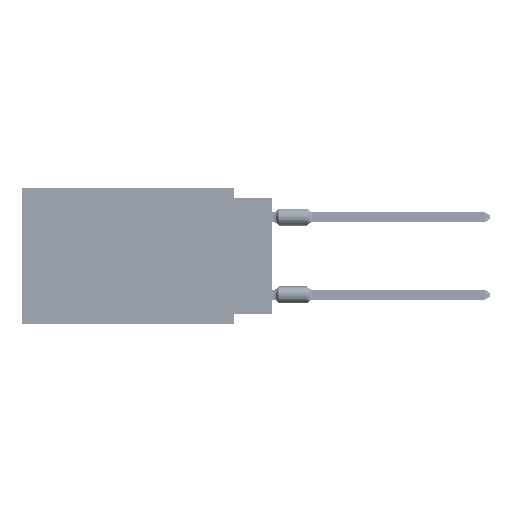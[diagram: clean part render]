
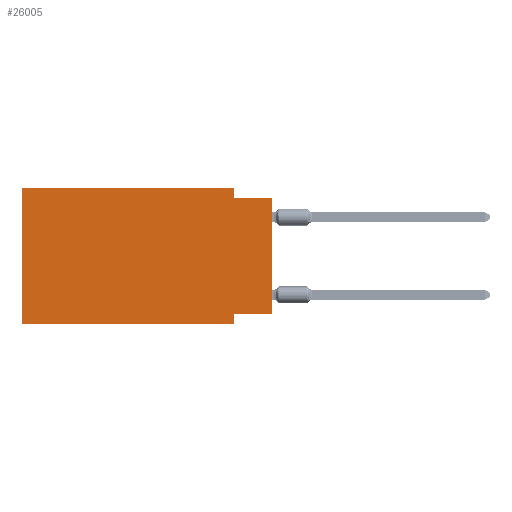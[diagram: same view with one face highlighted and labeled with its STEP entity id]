
A CAD part, left-side view. The second image highlights one B-rep face of the part: STEP entity #26005.
In plain terms, the highlighted planar face has unit normal (-1, 0, 0).
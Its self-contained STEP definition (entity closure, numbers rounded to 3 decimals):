
#1491 = VECTOR ( 'NONE', #83403, 1000. ) ;
#2519 = EDGE_CURVE ( 'NONE', #63819, #56504, #34661, .T. ) ;
#3334 = DIRECTION ( 'NONE',  ( 0., 0., -1. ) ) ;
#5311 = EDGE_CURVE ( 'NONE', #20957, #39904, #30329, .T. ) ;
#7591 = ORIENTED_EDGE ( 'NONE', *, *, #12461, .F. ) ;
#8471 = EDGE_CURVE ( 'NONE', #83705, #11104, #82508, .T. ) ;
#8855 = VECTOR ( 'NONE', #21555, 1000. ) ;
#9452 = DIRECTION ( 'NONE',  ( 0., 1., 0. ) ) ;
#11104 = VERTEX_POINT ( 'NONE', #35772 ) ;
#12461 = EDGE_CURVE ( 'NONE', #27926, #83705, #72951, .T. ) ;
#20957 = VERTEX_POINT ( 'NONE', #21303 ) ;
#21303 = CARTESIAN_POINT ( 'NONE',  ( 0., 16.383, -8.89 ) ) ;
#21555 = DIRECTION ( 'NONE',  ( 0., -1., 0. ) ) ;
#21597 = DIRECTION ( 'NONE',  ( 0., -1., 0. ) ) ;
#24676 = CARTESIAN_POINT ( 'NONE',  ( 0., 2.54, 0. ) ) ;
#26005 = ADVANCED_FACE ( 'NONE', ( #72023 ), #39058, .F. ) ;
#26928 = VECTOR ( 'NONE', #9452, 1000. ) ;
#27371 = VECTOR ( 'NONE', #74568, 1000. ) ;
#27926 = VERTEX_POINT ( 'NONE', #77089 ) ;
#29861 = CARTESIAN_POINT ( 'NONE',  ( 0., 2.54, 0. ) ) ;
#30329 = LINE ( 'NONE', #62856, #1491 ) ;
#31702 = CARTESIAN_POINT ( 'NONE',  ( 0., 0., -8.255 ) ) ;
#32203 = CARTESIAN_POINT ( 'NONE',  ( 0., 16.383, 0. ) ) ;
#33163 = CARTESIAN_POINT ( 'NONE',  ( 0., 16.383, 0. ) ) ;
#33397 = CARTESIAN_POINT ( 'NONE',  ( 0., 0., 0. ) ) ;
#33592 = LINE ( 'NONE', #54132, #62811 ) ;
#34661 = LINE ( 'NONE', #33397, #43506 ) ;
#35772 = CARTESIAN_POINT ( 'NONE',  ( 0., 2.54, -0.635 ) ) ;
#36086 = ORIENTED_EDGE ( 'NONE', *, *, #5311, .T. ) ;
#39058 = PLANE ( 'NONE',  #83180 ) ;
#39383 = ORIENTED_EDGE ( 'NONE', *, *, #8471, .F. ) ;
#39904 = VERTEX_POINT ( 'NONE', #80222 ) ;
#40854 = DIRECTION ( 'NONE',  ( 0., 0., 1. ) ) ;
#41967 = LINE ( 'NONE', #68087, #26928 ) ;
#42954 = ORIENTED_EDGE ( 'NONE', *, *, #81135, .F. ) ;
#43506 = VECTOR ( 'NONE', #73633, 1000. ) ;
#47248 = CARTESIAN_POINT ( 'NONE',  ( 0., 16.383, 0. ) ) ;
#48449 = CARTESIAN_POINT ( 'NONE',  ( 0., 2.54, -8.89 ) ) ;
#48486 = ORIENTED_EDGE ( 'NONE', *, *, #2519, .T. ) ;
#49396 = CARTESIAN_POINT ( 'NONE',  ( 0., 2.54, -8.255 ) ) ;
#51330 = ORIENTED_EDGE ( 'NONE', *, *, #63699, .F. ) ;
#51499 = ORIENTED_EDGE ( 'NONE', *, *, #62434, .F. ) ;
#54132 = CARTESIAN_POINT ( 'NONE',  ( 0., 0., -0.635 ) ) ;
#55719 = LINE ( 'NONE', #48449, #27371 ) ;
#56504 = VERTEX_POINT ( 'NONE', #77900 ) ;
#58322 = DIRECTION ( 'NONE',  ( 1., 0., 0. ) ) ;
#59396 = VECTOR ( 'NONE', #40854, 1000. ) ;
#62434 = EDGE_CURVE ( 'NONE', #11104, #56504, #33592, .T. ) ;
#62811 = VECTOR ( 'NONE', #21597, 1000. ) ;
#62856 = CARTESIAN_POINT ( 'NONE',  ( 0., 16.383, -8.89 ) ) ;
#63610 = VECTOR ( 'NONE', #3334, 1000. ) ;
#63699 = EDGE_CURVE ( 'NONE', #74128, #39904, #55719, .T. ) ;
#63819 = VERTEX_POINT ( 'NONE', #31702 ) ;
#67151 = ORIENTED_EDGE ( 'NONE', *, *, #68736, .F. ) ;
#68087 = CARTESIAN_POINT ( 'NONE',  ( 0., 0., -8.255 ) ) ;
#68736 = EDGE_CURVE ( 'NONE', #20957, #27926, #77279, .T. ) ;
#72023 = FACE_OUTER_BOUND ( 'NONE', #82361, .T. ) ;
#72951 = LINE ( 'NONE', #47248, #8855 ) ;
#73633 = DIRECTION ( 'NONE',  ( 0., 0., 1. ) ) ;
#74128 = VERTEX_POINT ( 'NONE', #49396 ) ;
#74568 = DIRECTION ( 'NONE',  ( 0., 0., -1. ) ) ;
#77089 = CARTESIAN_POINT ( 'NONE',  ( 0., 16.383, 0. ) ) ;
#77279 = LINE ( 'NONE', #33163, #59396 ) ;
#77900 = CARTESIAN_POINT ( 'NONE',  ( 0., 0., -0.635 ) ) ;
#80222 = CARTESIAN_POINT ( 'NONE',  ( 0., 2.54, -8.89 ) ) ;
#81135 = EDGE_CURVE ( 'NONE', #63819, #74128, #41967, .T. ) ;
#82361 = EDGE_LOOP ( 'NONE', ( #48486, #51499, #39383, #7591, #67151, #36086, #51330, #42954 ) ) ;
#82508 = LINE ( 'NONE', #24676, #63610 ) ;
#83180 = AXIS2_PLACEMENT_3D ( 'NONE', #32203, #58322, #84452 ) ;
#83403 = DIRECTION ( 'NONE',  ( 0., -1., 0. ) ) ;
#83705 = VERTEX_POINT ( 'NONE', #29861 ) ;
#84452 = DIRECTION ( 'NONE',  ( 0., 0., -1. ) ) ;
